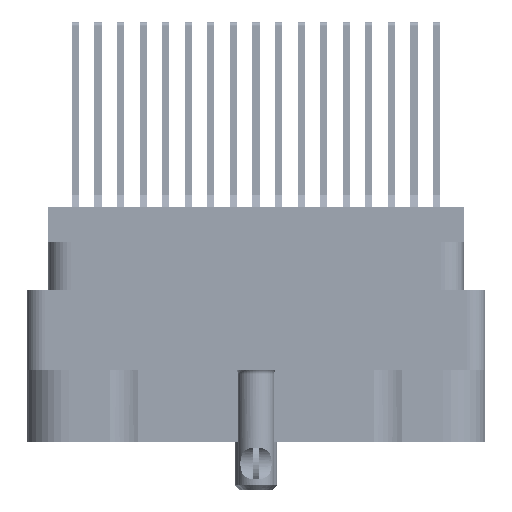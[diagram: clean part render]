
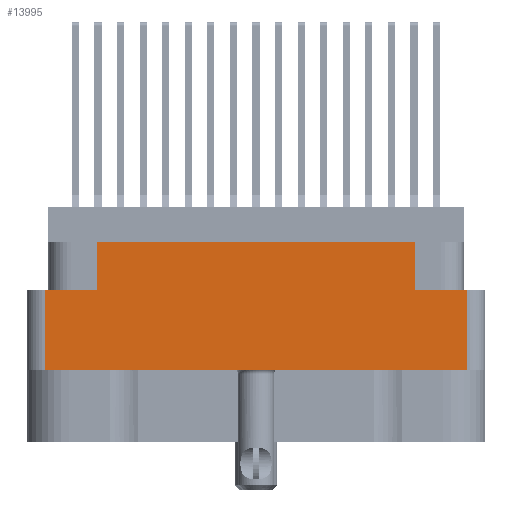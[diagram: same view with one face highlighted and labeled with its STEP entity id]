
A CAD part, left-side view. The second image highlights one B-rep face of the part: STEP entity #13995.
In plain terms, the highlighted planar face has unit normal (-1, 0, 0).
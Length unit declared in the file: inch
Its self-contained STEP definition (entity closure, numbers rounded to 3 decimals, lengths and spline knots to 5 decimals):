
#889 = LINE ( 'NONE', #17084, #9464 ) ;
#6543 = DIRECTION ( 'NONE',  ( 0., 0., 1. ) ) ;
#8780 = EDGE_LOOP ( 'NONE', ( #73192, #51938, #87036, #55215, #35395, #61971, #69320, #73946 ) ) ;
#9291 = VERTEX_POINT ( 'NONE', #63632 ) ;
#9464 = VECTOR ( 'NONE', #94779, 39.37008 ) ;
#9689 = VECTOR ( 'NONE', #21473, 39.37008 ) ;
#13045 = VECTOR ( 'NONE', #25348, 39.37008 ) ;
#13995 = ADVANCED_FACE ( 'NONE', ( #94230 ), #53310, .T. ) ;
#14814 = EDGE_CURVE ( 'NONE', #9291, #39100, #98814, .T. ) ;
#17084 = CARTESIAN_POINT ( 'NONE',  ( -1.375, 0.7625, -0.117 ) ) ;
#18163 = VERTEX_POINT ( 'NONE', #64694 ) ;
#20191 = CARTESIAN_POINT ( 'NONE',  ( -1.375, 0.7005, -0.274 ) ) ;
#20233 = DIRECTION ( 'NONE',  ( 0., -1., 0. ) ) ;
#20920 = CARTESIAN_POINT ( 'NONE',  ( -1.375, 0.5285, -0.274 ) ) ;
#21473 = DIRECTION ( 'NONE',  ( 0., 0., 1. ) ) ;
#23046 = VECTOR ( 'NONE', #75808, 39.37008 ) ;
#24809 = EDGE_CURVE ( 'NONE', #30169, #97330, #47389, .T. ) ;
#25348 = DIRECTION ( 'NONE',  ( 0., 0., -1. ) ) ;
#27298 = CARTESIAN_POINT ( 'NONE',  ( -1.375, -0.7005, -0.54 ) ) ;
#28766 = CARTESIAN_POINT ( 'NONE',  ( -1.375, -0.7005, -0.274 ) ) ;
#30169 = VERTEX_POINT ( 'NONE', #27298 ) ;
#32130 = EDGE_CURVE ( 'NONE', #41208, #18163, #68726, .T. ) ;
#35395 = ORIENTED_EDGE ( 'NONE', *, *, #60429, .F. ) ;
#36334 = CARTESIAN_POINT ( 'NONE',  ( -1.375, -0.7625, -0.78 ) ) ;
#37083 = CARTESIAN_POINT ( 'NONE',  ( -1.375, 0.5285, -0.117 ) ) ;
#39100 = VERTEX_POINT ( 'NONE', #77825 ) ;
#41146 = VECTOR ( 'NONE', #48475, 39.37008 ) ;
#41208 = VERTEX_POINT ( 'NONE', #20191 ) ;
#41719 = EDGE_CURVE ( 'NONE', #18163, #30169, #58357, .T. ) ;
#43694 = LINE ( 'NONE', #79651, #41146 ) ;
#45181 = DIRECTION ( 'NONE',  ( -1., 0., 0. ) ) ;
#45681 = VECTOR ( 'NONE', #20233, 39.37008 ) ;
#46569 = CARTESIAN_POINT ( 'NONE',  ( -1.375, 0.5285, -0.274 ) ) ;
#47389 = LINE ( 'NONE', #91316, #9689 ) ;
#48475 = DIRECTION ( 'NONE',  ( 0., -1., 0. ) ) ;
#50117 = DIRECTION ( 'NONE',  ( 0., 0., 1. ) ) ;
#51101 = CARTESIAN_POINT ( 'NONE',  ( -1.375, 0., -0.274 ) ) ;
#51938 = ORIENTED_EDGE ( 'NONE', *, *, #32130, .T. ) ;
#53310 = PLANE ( 'NONE',  #64057 ) ;
#55215 = ORIENTED_EDGE ( 'NONE', *, *, #24809, .T. ) ;
#56829 = EDGE_CURVE ( 'NONE', #41208, #99634, #43694, .T. ) ;
#58357 = LINE ( 'NONE', #100109, #80270 ) ;
#60429 = EDGE_CURVE ( 'NONE', #9291, #97330, #99143, .T. ) ;
#61971 = ORIENTED_EDGE ( 'NONE', *, *, #14814, .T. ) ;
#63632 = CARTESIAN_POINT ( 'NONE',  ( -1.375, -0.5285, -0.274 ) ) ;
#64057 = AXIS2_PLACEMENT_3D ( 'NONE', #36334, #45181, #6543 ) ;
#64540 = CARTESIAN_POINT ( 'NONE',  ( -1.375, -0.5285, -0.274 ) ) ;
#64694 = CARTESIAN_POINT ( 'NONE',  ( -1.375, 0.7005, -0.54 ) ) ;
#66159 = DIRECTION ( 'NONE',  ( 0., -1., 0. ) ) ;
#68726 = LINE ( 'NONE', #86750, #13045 ) ;
#69320 = ORIENTED_EDGE ( 'NONE', *, *, #95214, .F. ) ;
#73192 = ORIENTED_EDGE ( 'NONE', *, *, #56829, .F. ) ;
#73946 = ORIENTED_EDGE ( 'NONE', *, *, #89163, .F. ) ;
#75808 = DIRECTION ( 'NONE',  ( 0., 0., 1. ) ) ;
#77825 = CARTESIAN_POINT ( 'NONE',  ( -1.375, -0.5285, -0.117 ) ) ;
#79651 = CARTESIAN_POINT ( 'NONE',  ( -1.375, 0., -0.274 ) ) ;
#80270 = VECTOR ( 'NONE', #66159, 39.37008 ) ;
#86750 = CARTESIAN_POINT ( 'NONE',  ( -1.375, 0.7005, -0.78 ) ) ;
#87036 = ORIENTED_EDGE ( 'NONE', *, *, #41719, .T. ) ;
#89163 = EDGE_CURVE ( 'NONE', #99634, #91756, #89829, .T. ) ;
#89829 = LINE ( 'NONE', #20920, #23046 ) ;
#91316 = CARTESIAN_POINT ( 'NONE',  ( -1.375, -0.7005, -0.78 ) ) ;
#91458 = VECTOR ( 'NONE', #50117, 39.37008 ) ;
#91756 = VERTEX_POINT ( 'NONE', #37083 ) ;
#94230 = FACE_OUTER_BOUND ( 'NONE', #8780, .T. ) ;
#94779 = DIRECTION ( 'NONE',  ( 0., -1., 0. ) ) ;
#95214 = EDGE_CURVE ( 'NONE', #91756, #39100, #889, .T. ) ;
#97330 = VERTEX_POINT ( 'NONE', #28766 ) ;
#98814 = LINE ( 'NONE', #64540, #91458 ) ;
#99143 = LINE ( 'NONE', #51101, #45681 ) ;
#99634 = VERTEX_POINT ( 'NONE', #46569 ) ;
#100109 = CARTESIAN_POINT ( 'NONE',  ( -1.375, 0., -0.54 ) ) ;
